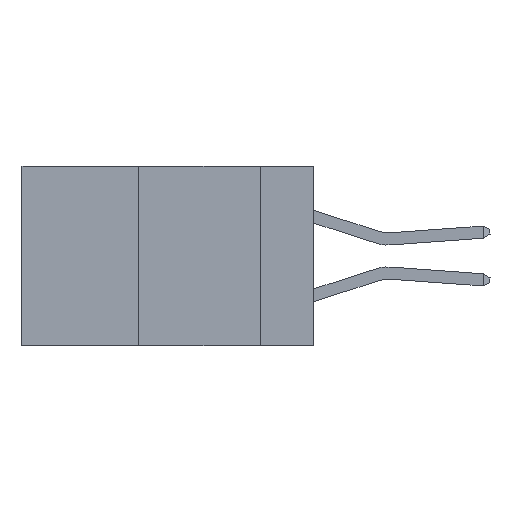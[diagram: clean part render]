
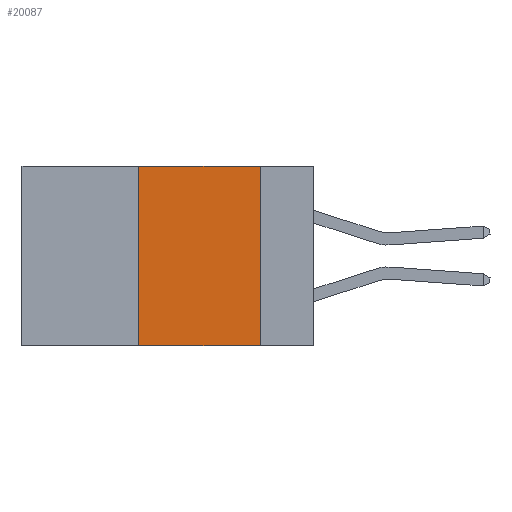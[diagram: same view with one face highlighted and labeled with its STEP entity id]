
A CAD part, left-side view. The second image highlights one B-rep face of the part: STEP entity #20087.
In plain terms, the highlighted planar face has unit normal (-1, 0, 0).
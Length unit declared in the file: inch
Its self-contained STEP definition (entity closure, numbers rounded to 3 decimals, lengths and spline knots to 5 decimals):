
#393 = CARTESIAN_POINT ( 'NONE',  ( 0., 0.36, -0.37 ) ) ;
#1341 = EDGE_CURVE ( 'NONE', #12979, #9363, #25034, .T. ) ;
#1774 = DIRECTION ( 'NONE',  ( 0., 0., 1. ) ) ;
#2562 = DIRECTION ( 'NONE',  ( 0., -1., 0. ) ) ;
#2683 = EDGE_CURVE ( 'NONE', #31553, #9363, #32500, .T. ) ;
#4582 = EDGE_CURVE ( 'NONE', #31553, #25104, #10676, .T. ) ;
#6809 = ORIENTED_EDGE ( 'NONE', *, *, #4582, .F. ) ;
#9264 = CARTESIAN_POINT ( 'NONE',  ( 0., 0.6, 0. ) ) ;
#9363 = VERTEX_POINT ( 'NONE', #26588 ) ;
#9370 = VECTOR ( 'NONE', #15761, 39.37008 ) ;
#10248 = CARTESIAN_POINT ( 'NONE',  ( 0., 0.11, 0. ) ) ;
#10676 = LINE ( 'NONE', #25988, #27346 ) ;
#12179 = DIRECTION ( 'NONE',  ( 1., 0., 0. ) ) ;
#12979 = VERTEX_POINT ( 'NONE', #31866 ) ;
#12992 = CARTESIAN_POINT ( 'NONE',  ( 0., 0.6, 0. ) ) ;
#13049 = DIRECTION ( 'NONE',  ( 0., 0., -1. ) ) ;
#13139 = EDGE_LOOP ( 'NONE', ( #13542, #14311, #6809, #24414 ) ) ;
#13542 = ORIENTED_EDGE ( 'NONE', *, *, #1341, .F. ) ;
#13569 = LINE ( 'NONE', #12992, #9370 ) ;
#13810 = FACE_OUTER_BOUND ( 'NONE', #13139, .T. ) ;
#14311 = ORIENTED_EDGE ( 'NONE', *, *, #34483, .F. ) ;
#14620 = DIRECTION ( 'NONE',  ( 0., 0., -1. ) ) ;
#14836 = CARTESIAN_POINT ( 'NONE',  ( 0., 0.36, 0. ) ) ;
#14861 = PLANE ( 'NONE',  #26119 ) ;
#15761 = DIRECTION ( 'NONE',  ( 0., -1., 0. ) ) ;
#16675 = VECTOR ( 'NONE', #2562, 39.37008 ) ;
#17959 = VECTOR ( 'NONE', #13049, 39.37008 ) ;
#20087 = ADVANCED_FACE ( 'NONE', ( #13810 ), #14861, .F. ) ;
#24414 = ORIENTED_EDGE ( 'NONE', *, *, #2683, .T. ) ;
#25034 = LINE ( 'NONE', #10248, #17959 ) ;
#25104 = VERTEX_POINT ( 'NONE', #14836 ) ;
#25988 = CARTESIAN_POINT ( 'NONE',  ( 0., 0.36, 0. ) ) ;
#26119 = AXIS2_PLACEMENT_3D ( 'NONE', #9264, #12179, #14620 ) ;
#26588 = CARTESIAN_POINT ( 'NONE',  ( 0., 0.11, -0.37 ) ) ;
#27346 = VECTOR ( 'NONE', #1774, 39.37008 ) ;
#31553 = VERTEX_POINT ( 'NONE', #393 ) ;
#31866 = CARTESIAN_POINT ( 'NONE',  ( 0., 0.11, 0. ) ) ;
#32500 = LINE ( 'NONE', #33447, #16675 ) ;
#33447 = CARTESIAN_POINT ( 'NONE',  ( 0., 0.6, -0.37 ) ) ;
#34483 = EDGE_CURVE ( 'NONE', #25104, #12979, #13569, .T. ) ;
